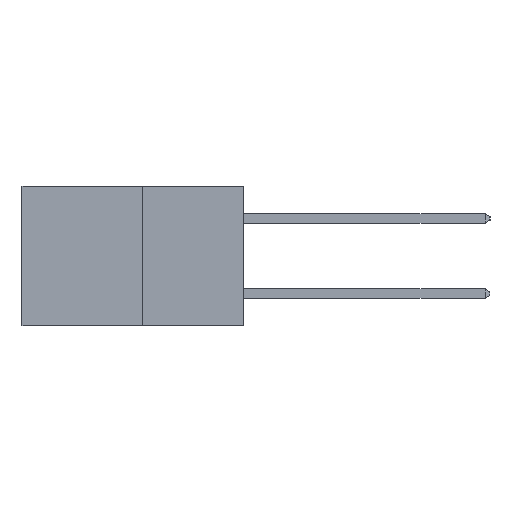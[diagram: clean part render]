
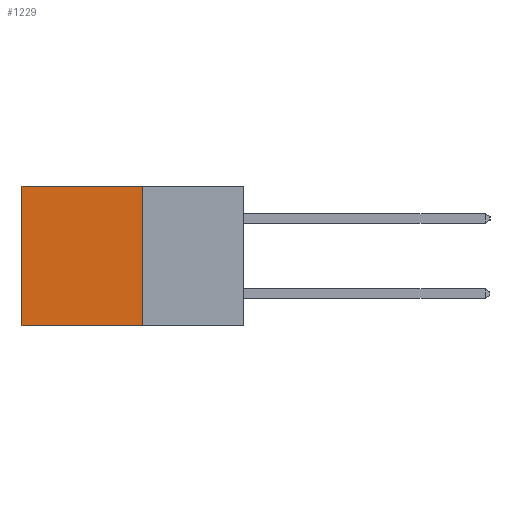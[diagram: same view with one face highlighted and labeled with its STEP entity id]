
A CAD part, left-side view. The second image highlights one B-rep face of the part: STEP entity #1229.
In plain terms, the highlighted planar face has unit normal (-1, 0, 0).
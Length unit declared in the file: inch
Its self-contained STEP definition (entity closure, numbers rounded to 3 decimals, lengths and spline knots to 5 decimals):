
#67 = VECTOR ( 'NONE', #1195, 39.37008 ) ;
#216 = FACE_OUTER_BOUND ( 'NONE', #2783, .T. ) ;
#592 = CARTESIAN_POINT ( 'NONE',  ( 0.277, 0.59, -0.37 ) ) ;
#616 = EDGE_CURVE ( 'NONE', #11249, #1417, #11409, .T. ) ;
#796 = VECTOR ( 'NONE', #10078, 39.37008 ) ;
#1012 = ORIENTED_EDGE ( 'NONE', *, *, #1049, .F. ) ;
#1049 = EDGE_CURVE ( 'NONE', #3878, #1417, #9835, .T. ) ;
#1195 = DIRECTION ( 'NONE',  ( 0., 1., 0. ) ) ;
#1229 = ADVANCED_FACE ( 'NONE', ( #216 ), #7928, .F. ) ;
#1417 = VERTEX_POINT ( 'NONE', #592 ) ;
#1860 = LINE ( 'NONE', #7008, #11579 ) ;
#2721 = CARTESIAN_POINT ( 'NONE',  ( 0.277, 0.27, -0.37 ) ) ;
#2783 = EDGE_LOOP ( 'NONE', ( #10759, #1012, #3549, #6060 ) ) ;
#3549 = ORIENTED_EDGE ( 'NONE', *, *, #5822, .F. ) ;
#3599 = CARTESIAN_POINT ( 'NONE',  ( 0.277, 0.59, -0.37 ) ) ;
#3770 = AXIS2_PLACEMENT_3D ( 'NONE', #10727, #11067, #10291 ) ;
#3878 = VERTEX_POINT ( 'NONE', #6324 ) ;
#5822 = EDGE_CURVE ( 'NONE', #8294, #3878, #1860, .T. ) ;
#5891 = CARTESIAN_POINT ( 'NONE',  ( 0.277, 0.59, 0. ) ) ;
#6060 = ORIENTED_EDGE ( 'NONE', *, *, #6726, .T. ) ;
#6132 = LINE ( 'NONE', #10239, #796 ) ;
#6324 = CARTESIAN_POINT ( 'NONE',  ( 0.277, 0.27, -0.37 ) ) ;
#6726 = EDGE_CURVE ( 'NONE', #8294, #11249, #6132, .T. ) ;
#6746 = VECTOR ( 'NONE', #9366, 39.37008 ) ;
#7008 = CARTESIAN_POINT ( 'NONE',  ( 0.277, 0.27, -0.37 ) ) ;
#7034 = DIRECTION ( 'NONE',  ( 0., 0., -1. ) ) ;
#7880 = CARTESIAN_POINT ( 'NONE',  ( 0.277, 0.27, 0. ) ) ;
#7928 = PLANE ( 'NONE',  #3770 ) ;
#8294 = VERTEX_POINT ( 'NONE', #7880 ) ;
#9366 = DIRECTION ( 'NONE',  ( 0., 0., -1. ) ) ;
#9835 = LINE ( 'NONE', #2721, #67 ) ;
#10078 = DIRECTION ( 'NONE',  ( 0., 1., 0. ) ) ;
#10239 = CARTESIAN_POINT ( 'NONE',  ( 0.277, 0.27, 0. ) ) ;
#10291 = DIRECTION ( 'NONE',  ( 0., 0., -1. ) ) ;
#10727 = CARTESIAN_POINT ( 'NONE',  ( 0.277, 0.27, -0.37 ) ) ;
#10759 = ORIENTED_EDGE ( 'NONE', *, *, #616, .T. ) ;
#11067 = DIRECTION ( 'NONE',  ( 1., 0., 0. ) ) ;
#11249 = VERTEX_POINT ( 'NONE', #5891 ) ;
#11409 = LINE ( 'NONE', #3599, #6746 ) ;
#11579 = VECTOR ( 'NONE', #7034, 39.37008 ) ;
